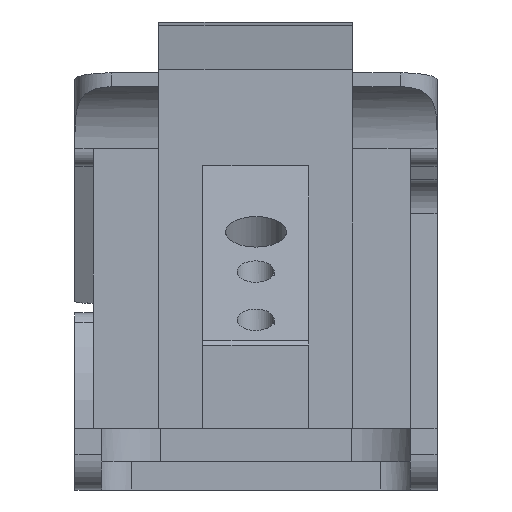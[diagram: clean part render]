
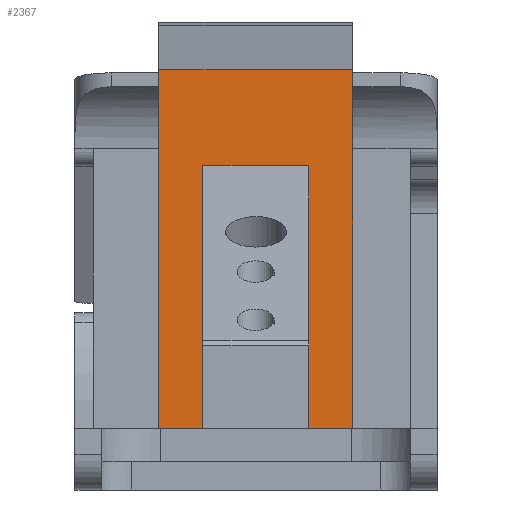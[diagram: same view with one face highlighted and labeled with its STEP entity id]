
A CAD part, left-side view. The second image highlights one B-rep face of the part: STEP entity #2367.
In plain terms, the highlighted planar face has unit normal (-1, 0, 0).
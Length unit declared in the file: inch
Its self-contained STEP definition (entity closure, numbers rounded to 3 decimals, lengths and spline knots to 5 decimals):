
#83=PLANE('',#2579);
#159=FACE_OUTER_BOUND('',#291,.T.);
#291=EDGE_LOOP('',(#1794,#1795,#1796,#1797,#1798,#1799,#1800,#1801));
#451=LINE('',#3663,#685);
#459=LINE('',#3695,#693);
#467=LINE('',#3727,#701);
#500=LINE('',#3882,#734);
#504=LINE('',#3890,#738);
#506=LINE('',#3893,#740);
#508=LINE('',#3897,#742);
#509=LINE('',#3898,#743);
#685=VECTOR('',#2888,0.3937);
#693=VECTOR('',#2916,0.3937);
#701=VECTOR('',#2944,0.3937);
#734=VECTOR('',#3033,0.3937);
#738=VECTOR('',#3043,0.3937);
#740=VECTOR('',#3045,0.3937);
#742=VECTOR('',#3049,0.3937);
#743=VECTOR('',#3050,0.3937);
#1043=VERTEX_POINT('',#3660);
#1044=VERTEX_POINT('',#3662);
#1057=VERTEX_POINT('',#3693);
#1058=VERTEX_POINT('',#3694);
#1107=VERTEX_POINT('',#3879);
#1108=VERTEX_POINT('',#3881);
#1110=VERTEX_POINT('',#3892);
#1111=VERTEX_POINT('',#3896);
#1290=EDGE_CURVE('',#1043,#1044,#451,.T.);
#1306=EDGE_CURVE('',#1057,#1058,#459,.T.);
#1323=EDGE_CURVE('',#1058,#1043,#467,.T.);
#1375=EDGE_CURVE('',#1108,#1107,#500,.T.);
#1379=EDGE_CURVE('',#1108,#1057,#504,.T.);
#1381=EDGE_CURVE('',#1110,#1044,#506,.T.);
#1383=EDGE_CURVE('',#1107,#1111,#508,.T.);
#1384=EDGE_CURVE('',#1111,#1110,#509,.T.);
#1794=ORIENTED_EDGE('',*,*,#1306,.F.);
#1795=ORIENTED_EDGE('',*,*,#1379,.F.);
#1796=ORIENTED_EDGE('',*,*,#1375,.T.);
#1797=ORIENTED_EDGE('',*,*,#1383,.T.);
#1798=ORIENTED_EDGE('',*,*,#1384,.T.);
#1799=ORIENTED_EDGE('',*,*,#1381,.T.);
#1800=ORIENTED_EDGE('',*,*,#1290,.F.);
#1801=ORIENTED_EDGE('',*,*,#1323,.F.);
#2367=ADVANCED_FACE('',(#159),#83,.T.);
#2579=AXIS2_PLACEMENT_3D('',#3895,#3047,#3048);
#2888=DIRECTION('',(0.,0.,-1.));
#2916=DIRECTION('',(0.,0.,1.));
#2944=DIRECTION('',(0.,-1.,0.));
#3033=DIRECTION('',(0.,0.,1.));
#3043=DIRECTION('',(0.,1.,0.));
#3045=DIRECTION('',(0.,-1.,0.));
#3047=DIRECTION('center_axis',(-1.,0.,0.));
#3048=DIRECTION('ref_axis',(0.,0.,-1.));
#3049=DIRECTION('',(0.,-1.,0.));
#3050=DIRECTION('',(0.,0.,-1.));
#3660=CARTESIAN_POINT('',(0.,-0.342,0.));
#3662=CARTESIAN_POINT('',(0.,-0.342,-1.2695));
#3663=CARTESIAN_POINT('',(0.,-0.342,-0.27478));
#3693=CARTESIAN_POINT('',(0.,0.344,-1.2695));
#3694=CARTESIAN_POINT('',(0.,0.344,0.));
#3695=CARTESIAN_POINT('',(0.,0.344,-0.2742));
#3727=CARTESIAN_POINT('',(0.,0.344,0.));
#3879=CARTESIAN_POINT('',(0.,0.1885,-0.3395));
#3881=CARTESIAN_POINT('',(0.,0.1885,-1.2695));
#3882=CARTESIAN_POINT('',(0.,0.1885,-0.45458));
#3890=CARTESIAN_POINT('',(0.,0.344,-1.2695));
#3892=CARTESIAN_POINT('',(0.,-0.1865,-1.2695));
#3893=CARTESIAN_POINT('',(0.,0.344,-1.2695));
#3895=CARTESIAN_POINT('Origin',(0.,0.344,0.));
#3896=CARTESIAN_POINT('',(0.,-0.1865,-0.3395));
#3897=CARTESIAN_POINT('',(0.,0.26625,-0.3395));
#3898=CARTESIAN_POINT('',(0.,-0.1865,-0.40225));
